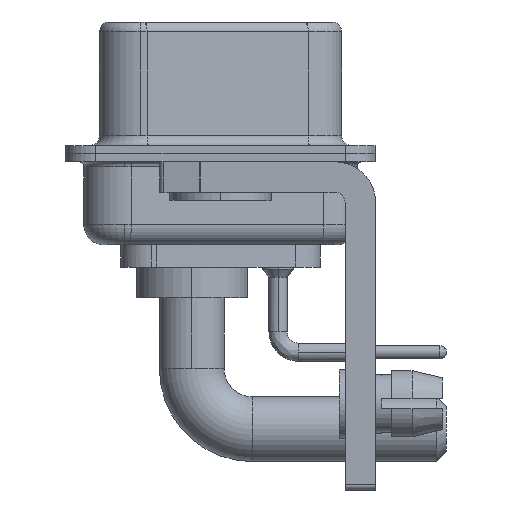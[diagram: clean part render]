
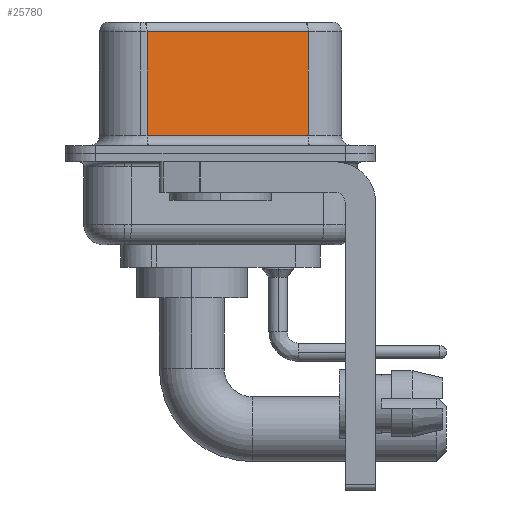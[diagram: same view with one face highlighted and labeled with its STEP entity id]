
A CAD part, left-side view. The second image highlights one B-rep face of the part: STEP entity #25780.
In plain terms, the highlighted planar face has unit normal (-0.985, -0.174, 0).
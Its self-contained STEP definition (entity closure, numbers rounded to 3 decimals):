
#198 = VERTEX_POINT ( 'NONE', #10425 ) ;
#1544 = FACE_OUTER_BOUND ( 'NONE', #13061, .T. ) ;
#1559 = VERTEX_POINT ( 'NONE', #3670 ) ;
#1925 = LINE ( 'NONE', #11736, #20690 ) ;
#2058 = EDGE_CURVE ( 'NONE', #3214, #198, #1925, .T. ) ;
#3214 = VERTEX_POINT ( 'NONE', #19468 ) ;
#3670 = CARTESIAN_POINT ( 'NONE',  ( 5.132, -4.322, 0.9 ) ) ;
#4102 = DIRECTION ( 'NONE',  ( 0., 0., -1. ) ) ;
#4683 = VECTOR ( 'NONE', #4102, 1000. ) ;
#5554 = ORIENTED_EDGE ( 'NONE', *, *, #6088, .T. ) ;
#6088 = EDGE_CURVE ( 'NONE', #21493, #1559, #14315, .T. ) ;
#7058 = ORIENTED_EDGE ( 'NONE', *, *, #17492, .F. ) ;
#7508 = CARTESIAN_POINT ( 'NONE',  ( 5.132, -4.322, 6.52 ) ) ;
#8095 = ORIENTED_EDGE ( 'NONE', *, *, #19695, .T. ) ;
#9882 = DIRECTION ( 'NONE',  ( -0.174, 0.985, 0. ) ) ;
#10306 = VECTOR ( 'NONE', #22903, 1000. ) ;
#10425 = CARTESIAN_POINT ( 'NONE',  ( 3.73, 3.628, 6.02 ) ) ;
#11627 = PLANE ( 'NONE',  #19332 ) ;
#11736 = CARTESIAN_POINT ( 'NONE',  ( 5.132, -4.322, 6.02 ) ) ;
#11923 = CARTESIAN_POINT ( 'NONE',  ( 5.132, -4.322, 0.9 ) ) ;
#13061 = EDGE_LOOP ( 'NONE', ( #7058, #25528, #8095, #5554 ) ) ;
#13913 = DIRECTION ( 'NONE',  ( 0.174, -0.985, 0. ) ) ;
#14315 = LINE ( 'NONE', #11923, #16215 ) ;
#16215 = VECTOR ( 'NONE', #13913, 1000. ) ;
#16470 = CARTESIAN_POINT ( 'NONE',  ( 5.132, -4.322, 6.52 ) ) ;
#17064 = LINE ( 'NONE', #24899, #10306 ) ;
#17492 = EDGE_CURVE ( 'NONE', #3214, #1559, #22453, .T. ) ;
#19332 = AXIS2_PLACEMENT_3D ( 'NONE', #7508, #19488, #21464 ) ;
#19468 = CARTESIAN_POINT ( 'NONE',  ( 5.132, -4.322, 6.02 ) ) ;
#19488 = DIRECTION ( 'NONE',  ( 0.985, 0.174, 0. ) ) ;
#19695 = EDGE_CURVE ( 'NONE', #198, #21493, #17064, .T. ) ;
#20690 = VECTOR ( 'NONE', #9882, 1000. ) ;
#21464 = DIRECTION ( 'NONE',  ( -0.174, 0.985, 0. ) ) ;
#21493 = VERTEX_POINT ( 'NONE', #22076 ) ;
#22076 = CARTESIAN_POINT ( 'NONE',  ( 3.73, 3.628, 0.9 ) ) ;
#22453 = LINE ( 'NONE', #16470, #4683 ) ;
#22903 = DIRECTION ( 'NONE',  ( 0., 0., -1. ) ) ;
#24899 = CARTESIAN_POINT ( 'NONE',  ( 3.73, 3.628, 6.52 ) ) ;
#25528 = ORIENTED_EDGE ( 'NONE', *, *, #2058, .T. ) ;
#25780 = ADVANCED_FACE ( 'NONE', ( #1544 ), #11627, .F. ) ;
